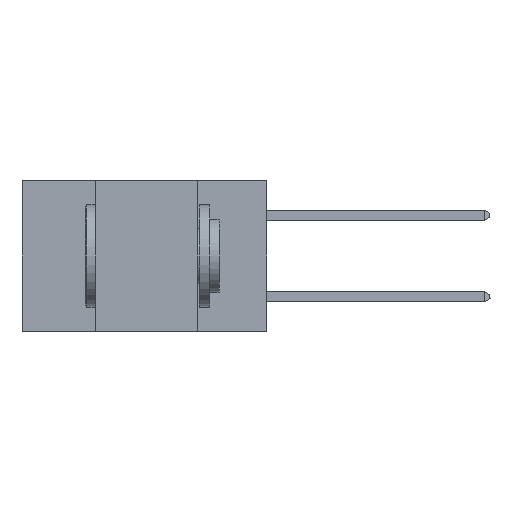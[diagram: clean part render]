
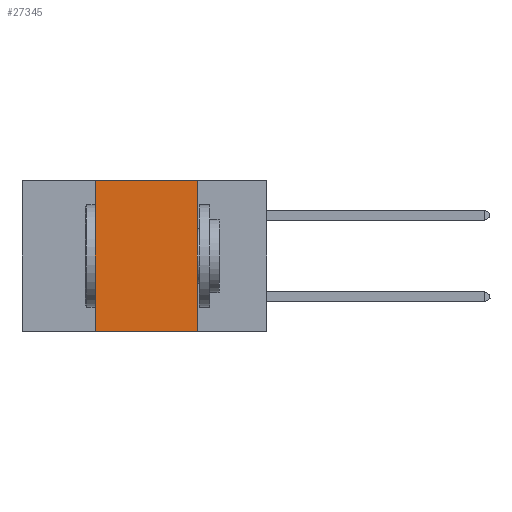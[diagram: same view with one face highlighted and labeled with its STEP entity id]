
A CAD part, left-side view. The second image highlights one B-rep face of the part: STEP entity #27345.
In plain terms, the highlighted planar face has unit normal (-1, 0, 0).
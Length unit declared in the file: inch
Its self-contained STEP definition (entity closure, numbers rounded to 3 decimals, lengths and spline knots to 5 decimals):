
#99 = EDGE_CURVE ( 'NONE', #6427, #4948, #4547, .T. ) ;
#176 = CARTESIAN_POINT ( 'NONE',  ( 0., 0.42, -0.37 ) ) ;
#365 = VECTOR ( 'NONE', #8875, 39.37008 ) ;
#996 = ORIENTED_EDGE ( 'NONE', *, *, #5260, .F. ) ;
#4075 = ORIENTED_EDGE ( 'NONE', *, *, #23617, .F. ) ;
#4437 = VERTEX_POINT ( 'NONE', #20790 ) ;
#4547 = LINE ( 'NONE', #21110, #11829 ) ;
#4948 = VERTEX_POINT ( 'NONE', #14794 ) ;
#5260 = EDGE_CURVE ( 'NONE', #6427, #4437, #7313, .T. ) ;
#5535 = ORIENTED_EDGE ( 'NONE', *, *, #13419, .F. ) ;
#6427 = VERTEX_POINT ( 'NONE', #176 ) ;
#7101 = CARTESIAN_POINT ( 'NONE',  ( 0., 0.6, 0. ) ) ;
#7313 = LINE ( 'NONE', #26529, #365 ) ;
#7884 = DIRECTION ( 'NONE',  ( 0., -1., 0. ) ) ;
#8332 = FACE_OUTER_BOUND ( 'NONE', #10288, .T. ) ;
#8875 = DIRECTION ( 'NONE',  ( 0., 0., 1. ) ) ;
#9044 = CARTESIAN_POINT ( 'NONE',  ( 0., 0.17, 0. ) ) ;
#10288 = EDGE_LOOP ( 'NONE', ( #4075, #5535, #996, #19141 ) ) ;
#10484 = CARTESIAN_POINT ( 'NONE',  ( 0., 0.17, 0. ) ) ;
#11829 = VECTOR ( 'NONE', #7884, 39.37008 ) ;
#12250 = PLANE ( 'NONE',  #26547 ) ;
#12826 = DIRECTION ( 'NONE',  ( 0., 0., -1. ) ) ;
#13419 = EDGE_CURVE ( 'NONE', #4437, #27024, #15429, .T. ) ;
#14794 = CARTESIAN_POINT ( 'NONE',  ( 0., 0.17, -0.37 ) ) ;
#15079 = DIRECTION ( 'NONE',  ( 0., 0., -1. ) ) ;
#15429 = LINE ( 'NONE', #7101, #28533 ) ;
#16756 = CARTESIAN_POINT ( 'NONE',  ( 0., 0.6, 0. ) ) ;
#17072 = VECTOR ( 'NONE', #15079, 39.37008 ) ;
#19141 = ORIENTED_EDGE ( 'NONE', *, *, #99, .T. ) ;
#20150 = LINE ( 'NONE', #10484, #17072 ) ;
#20488 = DIRECTION ( 'NONE',  ( 0., -1., 0. ) ) ;
#20790 = CARTESIAN_POINT ( 'NONE',  ( 0., 0.42, 0. ) ) ;
#21110 = CARTESIAN_POINT ( 'NONE',  ( 0., 0.6, -0.37 ) ) ;
#23617 = EDGE_CURVE ( 'NONE', #27024, #4948, #20150, .T. ) ;
#26529 = CARTESIAN_POINT ( 'NONE',  ( 0., 0.42, 0. ) ) ;
#26547 = AXIS2_PLACEMENT_3D ( 'NONE', #16756, #27644, #12826 ) ;
#27024 = VERTEX_POINT ( 'NONE', #9044 ) ;
#27345 = ADVANCED_FACE ( 'NONE', ( #8332 ), #12250, .F. ) ;
#27644 = DIRECTION ( 'NONE',  ( 1., 0., 0. ) ) ;
#28533 = VECTOR ( 'NONE', #20488, 39.37008 ) ;
